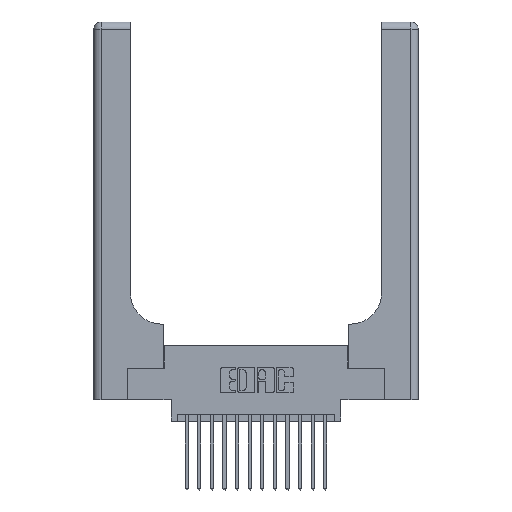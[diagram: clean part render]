
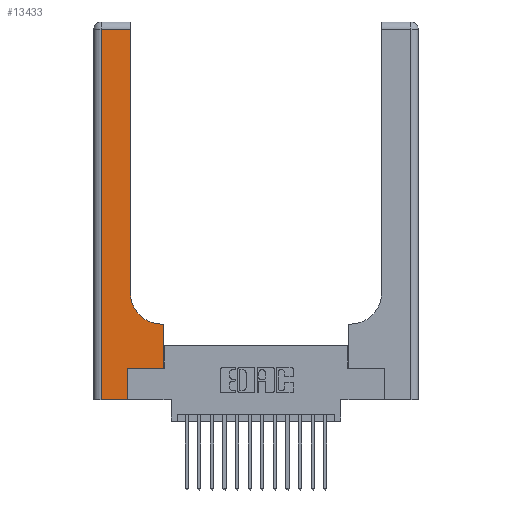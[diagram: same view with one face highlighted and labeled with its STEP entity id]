
A CAD part, top view. The second image highlights one B-rep face of the part: STEP entity #13433.
In plain terms, the highlighted planar face has unit normal (0, 0, 1).
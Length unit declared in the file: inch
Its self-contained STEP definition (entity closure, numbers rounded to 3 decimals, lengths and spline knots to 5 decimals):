
#343 = LINE ( 'NONE', #2234, #7621 ) ;
#891 = ORIENTED_EDGE ( 'NONE', *, *, #1595, .T. ) ;
#894 = CARTESIAN_POINT ( 'NONE',  ( 0.269, 0., 0.37 ) ) ;
#1128 = DIRECTION ( 'NONE',  ( 0., 1., 0. ) ) ;
#1157 = VERTEX_POINT ( 'NONE', #2761 ) ;
#1253 = CIRCLE ( 'NONE', #10807, 0.25 ) ;
#1288 = AXIS2_PLACEMENT_3D ( 'NONE', #4939, #15144, #3682 ) ;
#1595 = EDGE_CURVE ( 'NONE', #2493, #7822, #2232, .T. ) ;
#2055 = DIRECTION ( 'NONE',  ( 0., 1., 0. ) ) ;
#2126 = CARTESIAN_POINT ( 'NONE',  ( 0.5585, 0.25, 0.37 ) ) ;
#2205 = ORIENTED_EDGE ( 'NONE', *, *, #13017, .T. ) ;
#2232 = LINE ( 'NONE', #5332, #12008 ) ;
#2234 = CARTESIAN_POINT ( 'NONE',  ( 0., 0., 0.37 ) ) ;
#2293 = VERTEX_POINT ( 'NONE', #3568 ) ;
#2459 = DIRECTION ( 'NONE',  ( 0., -1., 0. ) ) ;
#2493 = VERTEX_POINT ( 'NONE', #17207 ) ;
#2761 = CARTESIAN_POINT ( 'NONE',  ( 0.5415, 0.6, 0.37 ) ) ;
#2783 = CARTESIAN_POINT ( 'NONE',  ( 0.269, 0., 0.37 ) ) ;
#2809 = CARTESIAN_POINT ( 'NONE',  ( 0.2915, 2.94, 0.37 ) ) ;
#3260 = ORIENTED_EDGE ( 'NONE', *, *, #18302, .T. ) ;
#3293 = VERTEX_POINT ( 'NONE', #16936 ) ;
#3306 = VERTEX_POINT ( 'NONE', #894 ) ;
#3313 = ORIENTED_EDGE ( 'NONE', *, *, #4347, .T. ) ;
#3527 = DIRECTION ( 'NONE',  ( 1., 0., 0. ) ) ;
#3567 = ORIENTED_EDGE ( 'NONE', *, *, #13854, .T. ) ;
#3568 = CARTESIAN_POINT ( 'NONE',  ( 0.269, 0.25, 0.37 ) ) ;
#3650 = CARTESIAN_POINT ( 'NONE',  ( 0.269, 0.25, 0.37 ) ) ;
#3682 = DIRECTION ( 'NONE',  ( -1., 0., 0. ) ) ;
#4209 = CARTESIAN_POINT ( 'NONE',  ( 0.5415, 0.85, 0.37 ) ) ;
#4347 = EDGE_CURVE ( 'NONE', #1157, #3293, #1253, .T. ) ;
#4349 = VECTOR ( 'NONE', #12102, 39.37008 ) ;
#4370 = EDGE_CURVE ( 'NONE', #15403, #1157, #8990, .T. ) ;
#4939 = CARTESIAN_POINT ( 'NONE',  ( 0., 3., 0.37 ) ) ;
#5101 = LINE ( 'NONE', #3650, #15083 ) ;
#5167 = DIRECTION ( 'NONE',  ( 1., 0., 0. ) ) ;
#5227 = CARTESIAN_POINT ( 'NONE',  ( 0.5585, 0.6, 0.37 ) ) ;
#5332 = CARTESIAN_POINT ( 'NONE',  ( 0.06, 3., 0.37 ) ) ;
#5651 = DIRECTION ( 'NONE',  ( 0., 0., -1. ) ) ;
#6149 = VERTEX_POINT ( 'NONE', #7834 ) ;
#6744 = VECTOR ( 'NONE', #10320, 39.37008 ) ;
#7595 = CARTESIAN_POINT ( 'NONE',  ( 0.2915, 3., 0.37 ) ) ;
#7621 = VECTOR ( 'NONE', #5167, 39.37008 ) ;
#7822 = VERTEX_POINT ( 'NONE', #8923 ) ;
#7834 = CARTESIAN_POINT ( 'NONE',  ( 0.5585, 0.25, 0.37 ) ) ;
#8327 = LINE ( 'NONE', #7595, #6744 ) ;
#8432 = ORIENTED_EDGE ( 'NONE', *, *, #4370, .T. ) ;
#8707 = DIRECTION ( 'NONE',  ( -1., 0., 0. ) ) ;
#8765 = EDGE_LOOP ( 'NONE', ( #14028, #3567, #891, #16846, #2205, #3260, #13256, #8432, #3313 ) ) ;
#8917 = LINE ( 'NONE', #2783, #11873 ) ;
#8923 = CARTESIAN_POINT ( 'NONE',  ( 0.06, 0., 0.37 ) ) ;
#8990 = LINE ( 'NONE', #13104, #10563 ) ;
#9542 = LINE ( 'NONE', #2126, #15887 ) ;
#10024 = LINE ( 'NONE', #13458, #4349 ) ;
#10320 = DIRECTION ( 'NONE',  ( 0., 1., 0. ) ) ;
#10563 = VECTOR ( 'NONE', #8707, 39.37008 ) ;
#10807 = AXIS2_PLACEMENT_3D ( 'NONE', #4209, #5651, #15800 ) ;
#11873 = VECTOR ( 'NONE', #1128, 39.37008 ) ;
#12008 = VECTOR ( 'NONE', #2459, 39.37008 ) ;
#12102 = DIRECTION ( 'NONE',  ( -1., 0., 0. ) ) ;
#12416 = VERTEX_POINT ( 'NONE', #2809 ) ;
#13017 = EDGE_CURVE ( 'NONE', #3306, #2293, #8917, .T. ) ;
#13104 = CARTESIAN_POINT ( 'NONE',  ( 0.2915, 0.6, 0.37 ) ) ;
#13256 = ORIENTED_EDGE ( 'NONE', *, *, #14713, .T. ) ;
#13433 = ADVANCED_FACE ( 'NONE', ( #15936 ), #18081, .F. ) ;
#13458 = CARTESIAN_POINT ( 'NONE',  ( 0., 2.94, 0.37 ) ) ;
#13854 = EDGE_CURVE ( 'NONE', #12416, #2493, #10024, .T. ) ;
#14028 = ORIENTED_EDGE ( 'NONE', *, *, #17436, .T. ) ;
#14713 = EDGE_CURVE ( 'NONE', #6149, #15403, #9542, .T. ) ;
#15083 = VECTOR ( 'NONE', #3527, 39.37008 ) ;
#15144 = DIRECTION ( 'NONE',  ( 0., 0., -1. ) ) ;
#15403 = VERTEX_POINT ( 'NONE', #5227 ) ;
#15800 = DIRECTION ( 'NONE',  ( 1., 0., 0. ) ) ;
#15887 = VECTOR ( 'NONE', #2055, 39.37008 ) ;
#15936 = FACE_OUTER_BOUND ( 'NONE', #8765, .T. ) ;
#16846 = ORIENTED_EDGE ( 'NONE', *, *, #17136, .T. ) ;
#16936 = CARTESIAN_POINT ( 'NONE',  ( 0.2915, 0.85, 0.37 ) ) ;
#17136 = EDGE_CURVE ( 'NONE', #7822, #3306, #343, .T. ) ;
#17207 = CARTESIAN_POINT ( 'NONE',  ( 0.06, 2.94, 0.37 ) ) ;
#17436 = EDGE_CURVE ( 'NONE', #3293, #12416, #8327, .T. ) ;
#18081 = PLANE ( 'NONE',  #1288 ) ;
#18302 = EDGE_CURVE ( 'NONE', #2293, #6149, #5101, .T. ) ;
